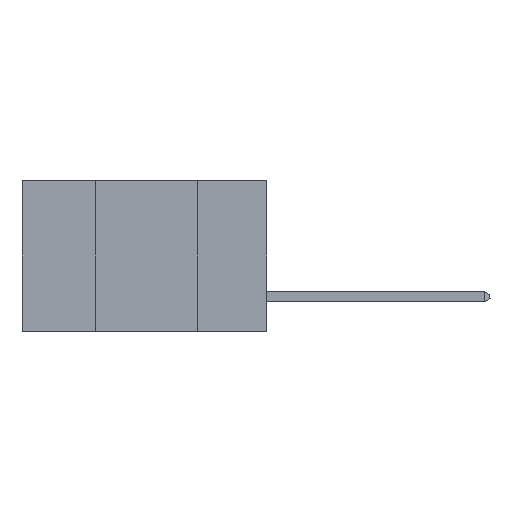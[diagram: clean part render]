
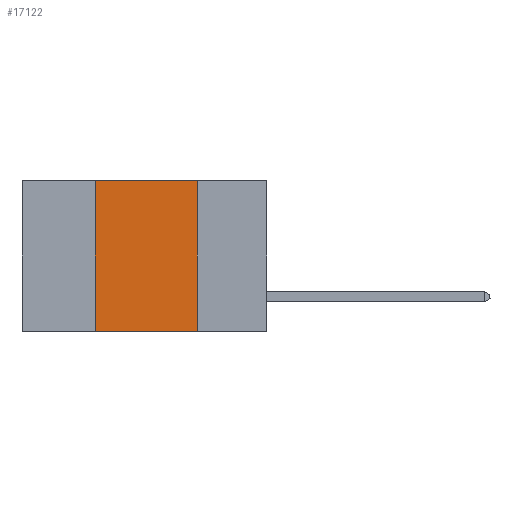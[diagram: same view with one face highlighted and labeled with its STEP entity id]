
A CAD part, left-side view. The second image highlights one B-rep face of the part: STEP entity #17122.
In plain terms, the highlighted planar face has unit normal (-1, 0, 0).
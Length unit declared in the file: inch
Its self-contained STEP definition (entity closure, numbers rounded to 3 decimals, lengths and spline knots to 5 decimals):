
#4538 = LINE ( 'NONE', #7527, #19678 ) ;
#6951 = VECTOR ( 'NONE', #34481, 39.37008 ) ;
#7475 = EDGE_CURVE ( 'NONE', #37745, #37086, #4538, .T. ) ;
#7527 = CARTESIAN_POINT ( 'NONE',  ( 0., 0.6, -0.37 ) ) ;
#9366 = CARTESIAN_POINT ( 'NONE',  ( 0., 0.17, 0. ) ) ;
#10050 = CARTESIAN_POINT ( 'NONE',  ( 0., 0.17, 0. ) ) ;
#10986 = PLANE ( 'NONE',  #28748 ) ;
#11263 = CARTESIAN_POINT ( 'NONE',  ( 0., 0.42, -0.37 ) ) ;
#11758 = ORIENTED_EDGE ( 'NONE', *, *, #13634, .F. ) ;
#13634 = EDGE_CURVE ( 'NONE', #37745, #43425, #33678, .T. ) ;
#13847 = DIRECTION ( 'NONE',  ( 0., 0., 1. ) ) ;
#15276 = VECTOR ( 'NONE', #35576, 39.37008 ) ;
#17122 = ADVANCED_FACE ( 'NONE', ( #39172 ), #10986, .F. ) ;
#19057 = DIRECTION ( 'NONE',  ( 1., 0., 0. ) ) ;
#19137 = CARTESIAN_POINT ( 'NONE',  ( 0., 0.42, 0. ) ) ;
#19678 = VECTOR ( 'NONE', #30229, 39.37008 ) ;
#21996 = VECTOR ( 'NONE', #13847, 39.37008 ) ;
#22338 = CARTESIAN_POINT ( 'NONE',  ( 0., 0.6, 0. ) ) ;
#23383 = EDGE_CURVE ( 'NONE', #43425, #45512, #35553, .T. ) ;
#28090 = CARTESIAN_POINT ( 'NONE',  ( 0., 0.42, 0. ) ) ;
#28748 = AXIS2_PLACEMENT_3D ( 'NONE', #33980, #19057, #37753 ) ;
#29412 = CARTESIAN_POINT ( 'NONE',  ( 0., 0.17, -0.37 ) ) ;
#30229 = DIRECTION ( 'NONE',  ( 0., -1., 0. ) ) ;
#33678 = LINE ( 'NONE', #19137, #21996 ) ;
#33980 = CARTESIAN_POINT ( 'NONE',  ( 0., 0.6, 0. ) ) ;
#34481 = DIRECTION ( 'NONE',  ( 0., -1., 0. ) ) ;
#35553 = LINE ( 'NONE', #22338, #6951 ) ;
#35576 = DIRECTION ( 'NONE',  ( 0., 0., -1. ) ) ;
#37086 = VERTEX_POINT ( 'NONE', #29412 ) ;
#37133 = EDGE_LOOP ( 'NONE', ( #41017, #45033, #11758, #47488 ) ) ;
#37745 = VERTEX_POINT ( 'NONE', #11263 ) ;
#37753 = DIRECTION ( 'NONE',  ( 0., 0., -1. ) ) ;
#39172 = FACE_OUTER_BOUND ( 'NONE', #37133, .T. ) ;
#41017 = ORIENTED_EDGE ( 'NONE', *, *, #46605, .F. ) ;
#43425 = VERTEX_POINT ( 'NONE', #28090 ) ;
#45033 = ORIENTED_EDGE ( 'NONE', *, *, #23383, .F. ) ;
#45512 = VERTEX_POINT ( 'NONE', #10050 ) ;
#46605 = EDGE_CURVE ( 'NONE', #45512, #37086, #47555, .T. ) ;
#47488 = ORIENTED_EDGE ( 'NONE', *, *, #7475, .T. ) ;
#47555 = LINE ( 'NONE', #9366, #15276 ) ;
